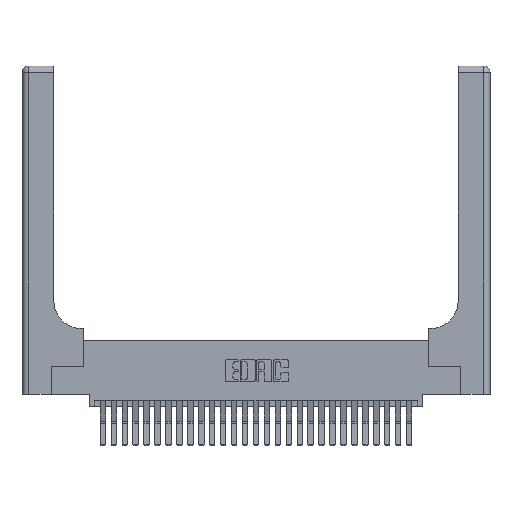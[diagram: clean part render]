
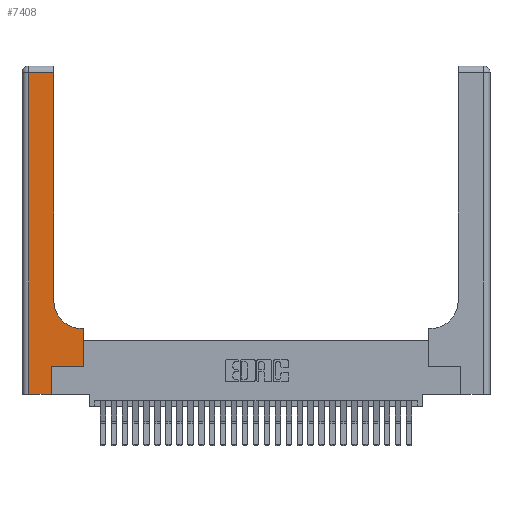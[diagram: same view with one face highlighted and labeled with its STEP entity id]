
A CAD part, top view. The second image highlights one B-rep face of the part: STEP entity #7408.
In plain terms, the highlighted planar face has unit normal (0, 0, 1).
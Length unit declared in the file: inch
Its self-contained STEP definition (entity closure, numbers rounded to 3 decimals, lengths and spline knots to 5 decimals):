
#685 = DIRECTION ( 'NONE',  ( -1., 0., 0. ) ) ;
#1080 = DIRECTION ( 'NONE',  ( -1., 0., 0. ) ) ;
#1282 = VERTEX_POINT ( 'NONE', #12677 ) ;
#1825 = VERTEX_POINT ( 'NONE', #29228 ) ;
#3184 = VERTEX_POINT ( 'NONE', #16075 ) ;
#3768 = VECTOR ( 'NONE', #17491, 39.37008 ) ;
#4487 = FACE_OUTER_BOUND ( 'NONE', #28106, .T. ) ;
#5212 = ORIENTED_EDGE ( 'NONE', *, *, #29318, .T. ) ;
#5603 = LINE ( 'NONE', #6852, #20046 ) ;
#5610 = DIRECTION ( 'NONE',  ( 0., 0., -1. ) ) ;
#5993 = DIRECTION ( 'NONE',  ( 0., 0., -1. ) ) ;
#6099 = CARTESIAN_POINT ( 'NONE',  ( 0.2915, 3., 0.37 ) ) ;
#6287 = VECTOR ( 'NONE', #685, 39.37008 ) ;
#6852 = CARTESIAN_POINT ( 'NONE',  ( 0.269, 0., 0.37 ) ) ;
#7151 = CARTESIAN_POINT ( 'NONE',  ( 0.269, 0.25, 0.37 ) ) ;
#7333 = EDGE_CURVE ( 'NONE', #1282, #3184, #14185, .T. ) ;
#7382 = EDGE_CURVE ( 'NONE', #27976, #29431, #29071, .T. ) ;
#7408 = ADVANCED_FACE ( 'NONE', ( #4487 ), #28577, .F. ) ;
#7839 = CARTESIAN_POINT ( 'NONE',  ( 0., 3., 0.37 ) ) ;
#7924 = VERTEX_POINT ( 'NONE', #9853 ) ;
#8107 = ORIENTED_EDGE ( 'NONE', *, *, #28473, .T. ) ;
#8919 = EDGE_CURVE ( 'NONE', #25766, #20544, #5603, .T. ) ;
#9569 = ORIENTED_EDGE ( 'NONE', *, *, #28614, .T. ) ;
#9785 = CARTESIAN_POINT ( 'NONE',  ( 0.269, 0., 0.37 ) ) ;
#9853 = CARTESIAN_POINT ( 'NONE',  ( 0.5585, 0.25, 0.37 ) ) ;
#10492 = CARTESIAN_POINT ( 'NONE',  ( 0.06, 3., 0.37 ) ) ;
#11464 = VECTOR ( 'NONE', #24690, 39.37008 ) ;
#11907 = EDGE_CURVE ( 'NONE', #1825, #27976, #26073, .T. ) ;
#12253 = CARTESIAN_POINT ( 'NONE',  ( 0.269, 0.25, 0.37 ) ) ;
#12677 = CARTESIAN_POINT ( 'NONE',  ( 0.06, 2.94, 0.37 ) ) ;
#13498 = DIRECTION ( 'NONE',  ( 0., -1., 0. ) ) ;
#14185 = LINE ( 'NONE', #10492, #20729 ) ;
#14569 = CARTESIAN_POINT ( 'NONE',  ( 0.2915, 0.6, 0.37 ) ) ;
#14868 = VECTOR ( 'NONE', #17191, 39.37008 ) ;
#14950 = DIRECTION ( 'NONE',  ( 0., 1., 0. ) ) ;
#15566 = DIRECTION ( 'NONE',  ( 1., 0., 0. ) ) ;
#15577 = CARTESIAN_POINT ( 'NONE',  ( 0., 0., 0.37 ) ) ;
#15678 = CARTESIAN_POINT ( 'NONE',  ( 0.5415, 0.85, 0.37 ) ) ;
#16075 = CARTESIAN_POINT ( 'NONE',  ( 0.06, 0., 0.37 ) ) ;
#16116 = VERTEX_POINT ( 'NONE', #18218 ) ;
#16349 = ORIENTED_EDGE ( 'NONE', *, *, #11907, .T. ) ;
#16418 = ORIENTED_EDGE ( 'NONE', *, *, #21308, .T. ) ;
#17032 = ORIENTED_EDGE ( 'NONE', *, *, #7333, .T. ) ;
#17155 = CARTESIAN_POINT ( 'NONE',  ( 0.2915, 0.85, 0.37 ) ) ;
#17191 = DIRECTION ( 'NONE',  ( 1., 0., 0. ) ) ;
#17486 = LINE ( 'NONE', #14569, #6287 ) ;
#17491 = DIRECTION ( 'NONE',  ( 0., 1., 0. ) ) ;
#17909 = ORIENTED_EDGE ( 'NONE', *, *, #7382, .T. ) ;
#18218 = CARTESIAN_POINT ( 'NONE',  ( 0.5585, 0.6, 0.37 ) ) ;
#19583 = ORIENTED_EDGE ( 'NONE', *, *, #21639, .T. ) ;
#19626 = LINE ( 'NONE', #20108, #3768 ) ;
#20046 = VECTOR ( 'NONE', #26476, 39.37008 ) ;
#20108 = CARTESIAN_POINT ( 'NONE',  ( 0.5585, 0.25, 0.37 ) ) ;
#20544 = VERTEX_POINT ( 'NONE', #7151 ) ;
#20729 = VECTOR ( 'NONE', #13498, 39.37008 ) ;
#21308 = EDGE_CURVE ( 'NONE', #29431, #1282, #24383, .T. ) ;
#21445 = VECTOR ( 'NONE', #23274, 39.37008 ) ;
#21639 = EDGE_CURVE ( 'NONE', #3184, #25766, #29201, .T. ) ;
#21835 = AXIS2_PLACEMENT_3D ( 'NONE', #15678, #5993, #15566 ) ;
#21899 = CARTESIAN_POINT ( 'NONE',  ( 0.2915, 2.94, 0.37 ) ) ;
#22876 = VECTOR ( 'NONE', #14950, 39.37008 ) ;
#23274 = DIRECTION ( 'NONE',  ( -1., 0., 0. ) ) ;
#23550 = LINE ( 'NONE', #12253, #14868 ) ;
#23910 = ORIENTED_EDGE ( 'NONE', *, *, #8919, .T. ) ;
#24383 = LINE ( 'NONE', #27801, #21445 ) ;
#24690 = DIRECTION ( 'NONE',  ( 1., 0., 0. ) ) ;
#25114 = AXIS2_PLACEMENT_3D ( 'NONE', #7839, #5610, #1080 ) ;
#25766 = VERTEX_POINT ( 'NONE', #9785 ) ;
#26073 = CIRCLE ( 'NONE', #21835, 0.25 ) ;
#26476 = DIRECTION ( 'NONE',  ( 0., 1., 0. ) ) ;
#27801 = CARTESIAN_POINT ( 'NONE',  ( 0., 2.94, 0.37 ) ) ;
#27976 = VERTEX_POINT ( 'NONE', #17155 ) ;
#28106 = EDGE_LOOP ( 'NONE', ( #17909, #16418, #17032, #19583, #23910, #5212, #8107, #9569, #16349 ) ) ;
#28473 = EDGE_CURVE ( 'NONE', #7924, #16116, #19626, .T. ) ;
#28577 = PLANE ( 'NONE',  #25114 ) ;
#28614 = EDGE_CURVE ( 'NONE', #16116, #1825, #17486, .T. ) ;
#29071 = LINE ( 'NONE', #6099, #22876 ) ;
#29201 = LINE ( 'NONE', #15577, #11464 ) ;
#29228 = CARTESIAN_POINT ( 'NONE',  ( 0.5415, 0.6, 0.37 ) ) ;
#29318 = EDGE_CURVE ( 'NONE', #20544, #7924, #23550, .T. ) ;
#29431 = VERTEX_POINT ( 'NONE', #21899 ) ;
